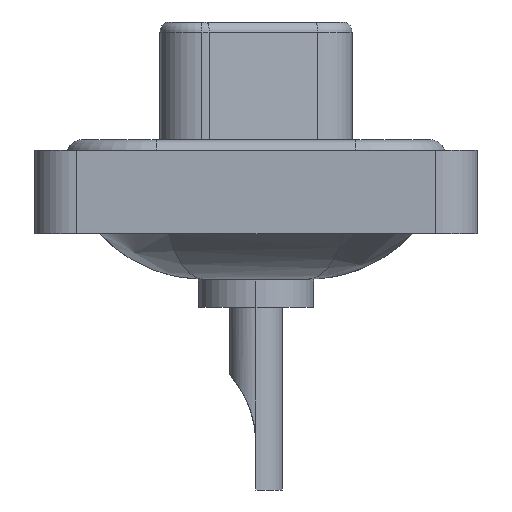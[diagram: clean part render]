
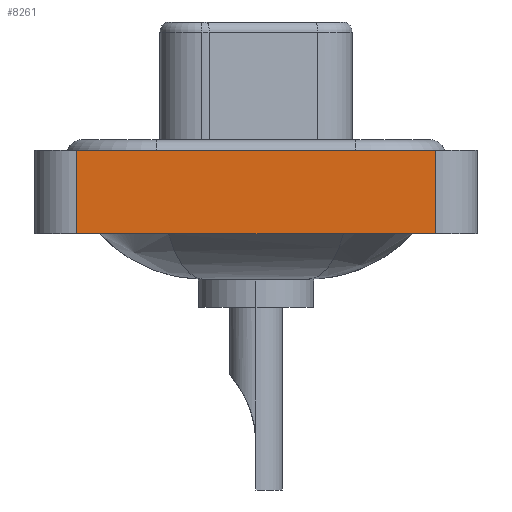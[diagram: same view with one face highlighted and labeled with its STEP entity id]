
A CAD part, left-side view. The second image highlights one B-rep face of the part: STEP entity #8261.
In plain terms, the highlighted planar face has unit normal (-1, 0, 0).
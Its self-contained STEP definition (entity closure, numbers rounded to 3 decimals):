
#224 = VECTOR ( 'NONE', #15329, 1000. ) ;
#467 = VERTEX_POINT ( 'NONE', #10523 ) ;
#1206 = CARTESIAN_POINT ( 'NONE',  ( -7.3, -8.55, -3.6 ) ) ;
#3808 = AXIS2_PLACEMENT_3D ( 'NONE', #3944, #16613, #7694 ) ;
#3944 = CARTESIAN_POINT ( 'NONE',  ( -7.3, -8.55, -3.6 ) ) ;
#4594 = CARTESIAN_POINT ( 'NONE',  ( -7.3, -8.55, 0.4 ) ) ;
#5580 = ORIENTED_EDGE ( 'NONE', *, *, #12962, .T. ) ;
#5728 = EDGE_LOOP ( 'NONE', ( #11963, #8941, #10691, #5580 ) ) ;
#6031 = CARTESIAN_POINT ( 'NONE',  ( -7.3, -8.55, -3.6 ) ) ;
#6040 = EDGE_CURVE ( 'NONE', #12059, #10203, #9001, .T. ) ;
#7034 = LINE ( 'NONE', #6031, #8832 ) ;
#7364 = CARTESIAN_POINT ( 'NONE',  ( -7.3, 8.55, 0.4 ) ) ;
#7524 = FACE_OUTER_BOUND ( 'NONE', #5728, .T. ) ;
#7694 = DIRECTION ( 'NONE',  ( 0., 0., 1. ) ) ;
#8261 = ADVANCED_FACE ( 'NONE', ( #7524 ), #15110, .T. ) ;
#8832 = VECTOR ( 'NONE', #10896, 1000. ) ;
#8941 = ORIENTED_EDGE ( 'NONE', *, *, #16300, .F. ) ;
#9001 = LINE ( 'NONE', #1206, #14484 ) ;
#10203 = VERTEX_POINT ( 'NONE', #11875 ) ;
#10273 = LINE ( 'NONE', #14141, #224 ) ;
#10523 = CARTESIAN_POINT ( 'NONE',  ( -7.3, 8.55, -3.6 ) ) ;
#10691 = ORIENTED_EDGE ( 'NONE', *, *, #11204, .F. ) ;
#10896 = DIRECTION ( 'NONE',  ( 0., -1., 0. ) ) ;
#11204 = EDGE_CURVE ( 'NONE', #467, #14773, #10273, .T. ) ;
#11875 = CARTESIAN_POINT ( 'NONE',  ( -7.3, -8.55, 0.4 ) ) ;
#11963 = ORIENTED_EDGE ( 'NONE', *, *, #6040, .T. ) ;
#12059 = VERTEX_POINT ( 'NONE', #12175 ) ;
#12175 = CARTESIAN_POINT ( 'NONE',  ( -7.3, -8.55, -3.6 ) ) ;
#12959 = VECTOR ( 'NONE', #13413, 1000. ) ;
#12962 = EDGE_CURVE ( 'NONE', #467, #12059, #7034, .T. ) ;
#13413 = DIRECTION ( 'NONE',  ( 0., -1., 0. ) ) ;
#14141 = CARTESIAN_POINT ( 'NONE',  ( -7.3, 8.55, -3.6 ) ) ;
#14484 = VECTOR ( 'NONE', #15311, 1000. ) ;
#14773 = VERTEX_POINT ( 'NONE', #7364 ) ;
#14837 = LINE ( 'NONE', #4594, #12959 ) ;
#15110 = PLANE ( 'NONE',  #3808 ) ;
#15311 = DIRECTION ( 'NONE',  ( 0., 0., 1. ) ) ;
#15329 = DIRECTION ( 'NONE',  ( 0., 0., 1. ) ) ;
#16300 = EDGE_CURVE ( 'NONE', #14773, #10203, #14837, .T. ) ;
#16613 = DIRECTION ( 'NONE',  ( -1., 0., 0. ) ) ;
